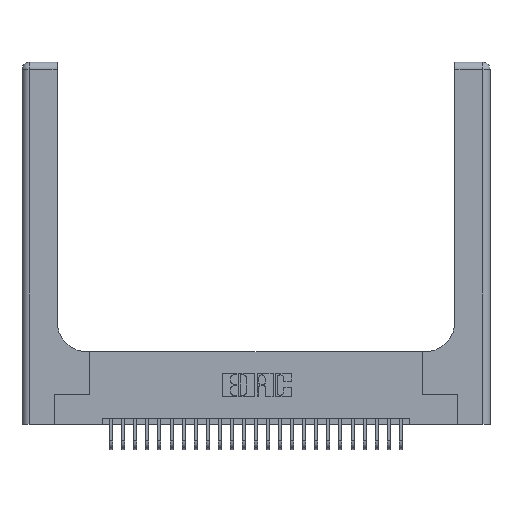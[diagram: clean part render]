
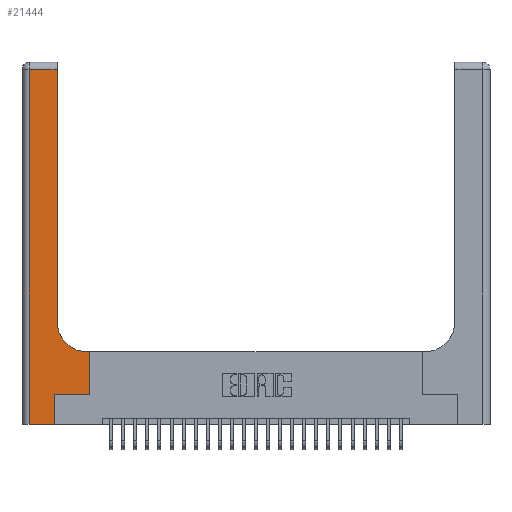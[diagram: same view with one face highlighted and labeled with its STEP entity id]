
A CAD part, top view. The second image highlights one B-rep face of the part: STEP entity #21444.
In plain terms, the highlighted planar face has unit normal (0, 0, 1).
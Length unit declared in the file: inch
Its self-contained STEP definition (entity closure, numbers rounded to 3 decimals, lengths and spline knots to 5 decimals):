
#528 = CARTESIAN_POINT ( 'NONE',  ( 0.06, 2.94, 0.37 ) ) ;
#766 = EDGE_CURVE ( 'NONE', #25373, #21274, #1983, .T. ) ;
#1514 = CARTESIAN_POINT ( 'NONE',  ( 0.2915, 0.6, 0.37 ) ) ;
#1983 = LINE ( 'NONE', #4648, #19071 ) ;
#2029 = EDGE_CURVE ( 'NONE', #20726, #12705, #10687, .T. ) ;
#2512 = VECTOR ( 'NONE', #12188, 39.37008 ) ;
#2912 = DIRECTION ( 'NONE',  ( 0., -1., 0. ) ) ;
#3887 = ORIENTED_EDGE ( 'NONE', *, *, #24260, .T. ) ;
#4604 = VECTOR ( 'NONE', #2912, 39.37008 ) ;
#4607 = ORIENTED_EDGE ( 'NONE', *, *, #16244, .T. ) ;
#4648 = CARTESIAN_POINT ( 'NONE',  ( 0.269, 0., 0.37 ) ) ;
#4739 = DIRECTION ( 'NONE',  ( 0., 1., 0. ) ) ;
#4861 = ORIENTED_EDGE ( 'NONE', *, *, #27259, .T. ) ;
#4960 = ORIENTED_EDGE ( 'NONE', *, *, #8816, .T. ) ;
#5387 = ORIENTED_EDGE ( 'NONE', *, *, #766, .T. ) ;
#5421 = CARTESIAN_POINT ( 'NONE',  ( 0.5585, 0.25, 0.37 ) ) ;
#5529 = CARTESIAN_POINT ( 'NONE',  ( 0., 2.94, 0.37 ) ) ;
#6085 = DIRECTION ( 'NONE',  ( 0., 1., 0. ) ) ;
#6130 = VERTEX_POINT ( 'NONE', #528 ) ;
#6232 = CARTESIAN_POINT ( 'NONE',  ( 0., 3., 0.37 ) ) ;
#6816 = VERTEX_POINT ( 'NONE', #12400 ) ;
#6830 = DIRECTION ( 'NONE',  ( 0., 0., -1. ) ) ;
#6872 = AXIS2_PLACEMENT_3D ( 'NONE', #6232, #8496, #23952 ) ;
#7089 = ORIENTED_EDGE ( 'NONE', *, *, #28098, .T. ) ;
#7599 = ORIENTED_EDGE ( 'NONE', *, *, #20796, .T. ) ;
#7832 = ORIENTED_EDGE ( 'NONE', *, *, #23951, .T. ) ;
#8159 = ORIENTED_EDGE ( 'NONE', *, *, #2029, .T. ) ;
#8352 = CARTESIAN_POINT ( 'NONE',  ( 0.2915, 0.85, 0.37 ) ) ;
#8496 = DIRECTION ( 'NONE',  ( 0., 0., -1. ) ) ;
#8816 = EDGE_CURVE ( 'NONE', #6816, #25373, #25546, .T. ) ;
#10687 = CIRCLE ( 'NONE', #13845, 0.25 ) ;
#10709 = LINE ( 'NONE', #11412, #21770 ) ;
#11412 = CARTESIAN_POINT ( 'NONE',  ( 0.2915, 3., 0.37 ) ) ;
#11431 = FACE_OUTER_BOUND ( 'NONE', #21169, .T. ) ;
#12128 = VERTEX_POINT ( 'NONE', #28379 ) ;
#12188 = DIRECTION ( 'NONE',  ( -1., 0., 0. ) ) ;
#12400 = CARTESIAN_POINT ( 'NONE',  ( 0.06, 0., 0.37 ) ) ;
#12508 = CARTESIAN_POINT ( 'NONE',  ( 0.2915, 2.94, 0.37 ) ) ;
#12628 = LINE ( 'NONE', #26042, #18509 ) ;
#12696 = DIRECTION ( 'NONE',  ( 1., 0., 0. ) ) ;
#12705 = VERTEX_POINT ( 'NONE', #8352 ) ;
#13151 = VECTOR ( 'NONE', #12696, 39.37008 ) ;
#13845 = AXIS2_PLACEMENT_3D ( 'NONE', #20156, #6830, #22363 ) ;
#15082 = DIRECTION ( 'NONE',  ( 1., 0., 0. ) ) ;
#15777 = LINE ( 'NONE', #22924, #4604 ) ;
#16244 = EDGE_CURVE ( 'NONE', #20205, #6130, #19606, .T. ) ;
#17110 = CARTESIAN_POINT ( 'NONE',  ( 0.5415, 0.6, 0.37 ) ) ;
#18509 = VECTOR ( 'NONE', #15082, 39.37008 ) ;
#19071 = VECTOR ( 'NONE', #20209, 39.37008 ) ;
#19353 = DIRECTION ( 'NONE',  ( -1., 0., 0. ) ) ;
#19560 = PLANE ( 'NONE',  #6872 ) ;
#19606 = LINE ( 'NONE', #5529, #2512 ) ;
#20156 = CARTESIAN_POINT ( 'NONE',  ( 0.5415, 0.85, 0.37 ) ) ;
#20205 = VERTEX_POINT ( 'NONE', #12508 ) ;
#20209 = DIRECTION ( 'NONE',  ( 0., 1., 0. ) ) ;
#20436 = CARTESIAN_POINT ( 'NONE',  ( 0.269, 0., 0.37 ) ) ;
#20726 = VERTEX_POINT ( 'NONE', #17110 ) ;
#20796 = EDGE_CURVE ( 'NONE', #28394, #12128, #27321, .T. ) ;
#21169 = EDGE_LOOP ( 'NONE', ( #3887, #4607, #4861, #4960, #5387, #7089, #7599, #7832, #8159 ) ) ;
#21274 = VERTEX_POINT ( 'NONE', #27553 ) ;
#21444 = ADVANCED_FACE ( 'NONE', ( #11431 ), #19560, .F. ) ;
#21615 = CARTESIAN_POINT ( 'NONE',  ( 0.5585, 0.25, 0.37 ) ) ;
#21770 = VECTOR ( 'NONE', #4739, 39.37008 ) ;
#21983 = LINE ( 'NONE', #1514, #22658 ) ;
#22363 = DIRECTION ( 'NONE',  ( 1., 0., 0. ) ) ;
#22658 = VECTOR ( 'NONE', #19353, 39.37008 ) ;
#22924 = CARTESIAN_POINT ( 'NONE',  ( 0.06, 3., 0.37 ) ) ;
#23951 = EDGE_CURVE ( 'NONE', #12128, #20726, #21983, .T. ) ;
#23952 = DIRECTION ( 'NONE',  ( -1., 0., 0. ) ) ;
#24260 = EDGE_CURVE ( 'NONE', #12705, #20205, #10709, .T. ) ;
#25373 = VERTEX_POINT ( 'NONE', #20436 ) ;
#25546 = LINE ( 'NONE', #27980, #13151 ) ;
#26042 = CARTESIAN_POINT ( 'NONE',  ( 0.269, 0.25, 0.37 ) ) ;
#26625 = VECTOR ( 'NONE', #6085, 39.37008 ) ;
#27259 = EDGE_CURVE ( 'NONE', #6130, #6816, #15777, .T. ) ;
#27321 = LINE ( 'NONE', #21615, #26625 ) ;
#27553 = CARTESIAN_POINT ( 'NONE',  ( 0.269, 0.25, 0.37 ) ) ;
#27980 = CARTESIAN_POINT ( 'NONE',  ( 0., 0., 0.37 ) ) ;
#28098 = EDGE_CURVE ( 'NONE', #21274, #28394, #12628, .T. ) ;
#28379 = CARTESIAN_POINT ( 'NONE',  ( 0.5585, 0.6, 0.37 ) ) ;
#28394 = VERTEX_POINT ( 'NONE', #5421 ) ;
